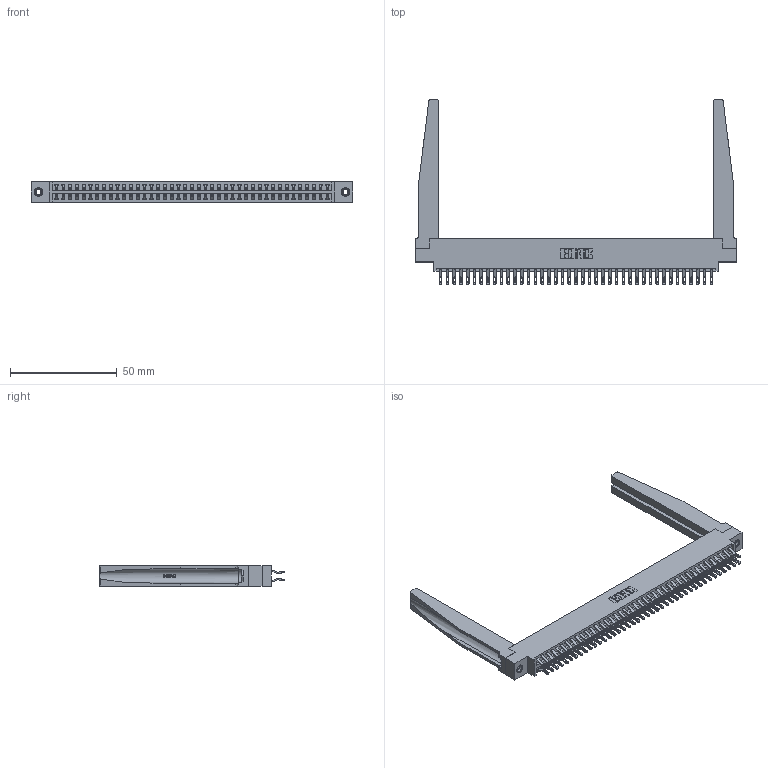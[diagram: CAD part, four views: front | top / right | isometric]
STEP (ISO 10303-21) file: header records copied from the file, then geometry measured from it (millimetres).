
FILE_DESCRIPTION (( 'STEP AP203' ), '1' );
FILE_NAME ('346-082-555-878.STEP', '2022-05-25T18:19:33', ( '' ), ( '' ), 'SwSTEP 2.0', 'SolidWorks 2020', '' );
FILE_SCHEMA (( 'CONFIG_CONTROL_DESIGN' ));
Length unit declared in the file: inch
Products named in the file (5): 346 Part_0.170 Offset - 0.156 Dia-TH; 345-292-001_555 Tail; 346-082-555-878; 346-220-078_345-220-078; 345-250-001_345-250-001-102
Assembly tree (87 placements, depth 2):
  346-082-555-878
    346 Part_0.170 Offset - 0.156 Dia-TH
    345-292-001_555 Tail  x82
    346-220-078_345-220-078  x2
    345-250-001_345-250-001-102  x2
Bounding box: 150.75 x 86.74 x 9.4 mm (x, y, z)
Volume: 21666.1 mm3; surface area: 27868.7 mm2
Topology: 87 solids, 87 shells, 5130 faces, 15991 edges, 10650 vertices
Faces by surface type: plane 2942, cylinder 2136, bspline 36, cone 12, torus 4
Entity records: 32514 total; most frequent: CARTESIAN_POINT 6339, ORIENTED_EDGE 5130, DIRECTION 4591, EDGE_CURVE 2565, VECTOR 2155, LINE 2155, VERTEX_POINT 1704, AXIS2_PLACEMENT_3D 1218
